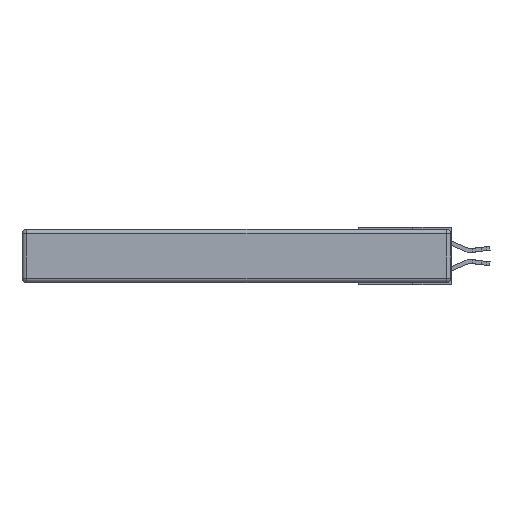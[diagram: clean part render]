
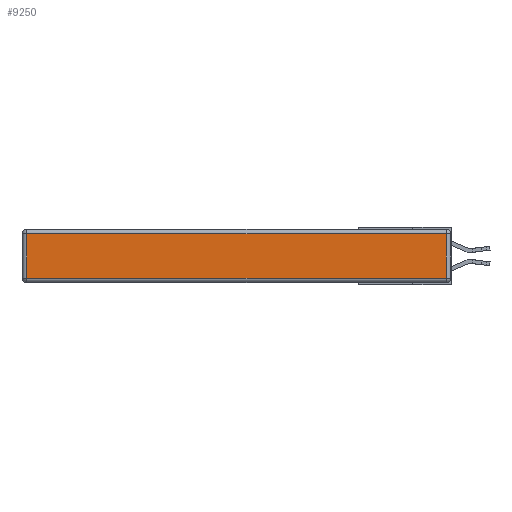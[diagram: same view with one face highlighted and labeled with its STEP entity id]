
A CAD part, left-side view. The second image highlights one B-rep face of the part: STEP entity #9250.
In plain terms, the highlighted planar face has unit normal (-1, 0, 0).
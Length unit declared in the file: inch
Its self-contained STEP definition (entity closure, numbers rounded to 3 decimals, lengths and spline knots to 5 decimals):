
#298 = LINE ( 'NONE', #4795, #12367 ) ;
#669 = LINE ( 'NONE', #13233, #6586 ) ;
#829 = LINE ( 'NONE', #2179, #11226 ) ;
#978 = DIRECTION ( 'NONE',  ( 0., 0., -1. ) ) ;
#1039 = VERTEX_POINT ( 'NONE', #1418 ) ;
#1230 = FACE_OUTER_BOUND ( 'NONE', #16341, .T. ) ;
#1264 = EDGE_CURVE ( 'NONE', #11712, #15201, #298, .T. ) ;
#1418 = CARTESIAN_POINT ( 'NONE',  ( 0., 2.72, -0.03 ) ) ;
#2179 = CARTESIAN_POINT ( 'NONE',  ( 0., 0.03, -0.343 ) ) ;
#2721 = LINE ( 'NONE', #6138, #10166 ) ;
#3192 = ORIENTED_EDGE ( 'NONE', *, *, #1264, .T. ) ;
#3505 = DIRECTION ( 'NONE',  ( 0., 0., 1. ) ) ;
#4795 = CARTESIAN_POINT ( 'NONE',  ( 0., 0., -0.313 ) ) ;
#5525 = CARTESIAN_POINT ( 'NONE',  ( 0., 0.03, -0.03 ) ) ;
#6138 = CARTESIAN_POINT ( 'NONE',  ( 0., 2.75, -0.03 ) ) ;
#6586 = VECTOR ( 'NONE', #978, 39.37008 ) ;
#8017 = ORIENTED_EDGE ( 'NONE', *, *, #13175, .T. ) ;
#8025 = CARTESIAN_POINT ( 'NONE',  ( 0., 0., -0.343 ) ) ;
#8068 = DIRECTION ( 'NONE',  ( 0., 0., 1. ) ) ;
#8988 = EDGE_CURVE ( 'NONE', #13970, #1039, #2721, .T. ) ;
#9250 = ADVANCED_FACE ( 'NONE', ( #1230 ), #11966, .T. ) ;
#9986 = AXIS2_PLACEMENT_3D ( 'NONE', #8025, #10966, #8068 ) ;
#10166 = VECTOR ( 'NONE', #10475, 39.37008 ) ;
#10475 = DIRECTION ( 'NONE',  ( 0., 1., 0. ) ) ;
#10966 = DIRECTION ( 'NONE',  ( -1., 0., 0. ) ) ;
#11028 = CARTESIAN_POINT ( 'NONE',  ( 0., 0.03, -0.313 ) ) ;
#11226 = VECTOR ( 'NONE', #3505, 39.37008 ) ;
#11712 = VERTEX_POINT ( 'NONE', #12947 ) ;
#11966 = PLANE ( 'NONE',  #9986 ) ;
#12367 = VECTOR ( 'NONE', #17118, 39.37008 ) ;
#12947 = CARTESIAN_POINT ( 'NONE',  ( 0., 2.72, -0.313 ) ) ;
#13175 = EDGE_CURVE ( 'NONE', #1039, #11712, #669, .T. ) ;
#13233 = CARTESIAN_POINT ( 'NONE',  ( 0., 2.72, -0.343 ) ) ;
#13970 = VERTEX_POINT ( 'NONE', #5525 ) ;
#14087 = EDGE_CURVE ( 'NONE', #15201, #13970, #829, .T. ) ;
#15201 = VERTEX_POINT ( 'NONE', #11028 ) ;
#16053 = ORIENTED_EDGE ( 'NONE', *, *, #14087, .T. ) ;
#16341 = EDGE_LOOP ( 'NONE', ( #3192, #16053, #17513, #8017 ) ) ;
#17118 = DIRECTION ( 'NONE',  ( 0., -1., 0. ) ) ;
#17513 = ORIENTED_EDGE ( 'NONE', *, *, #8988, .T. ) ;
